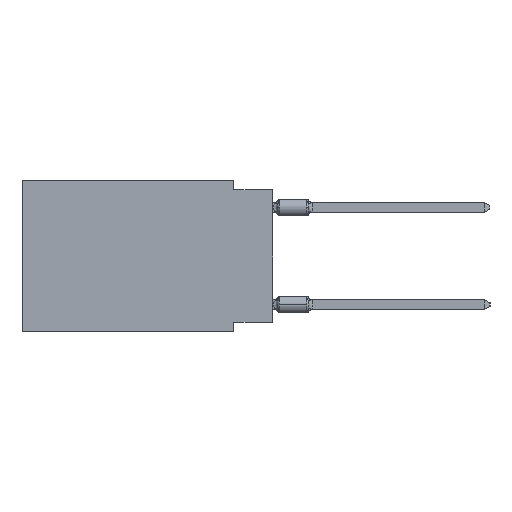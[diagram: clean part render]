
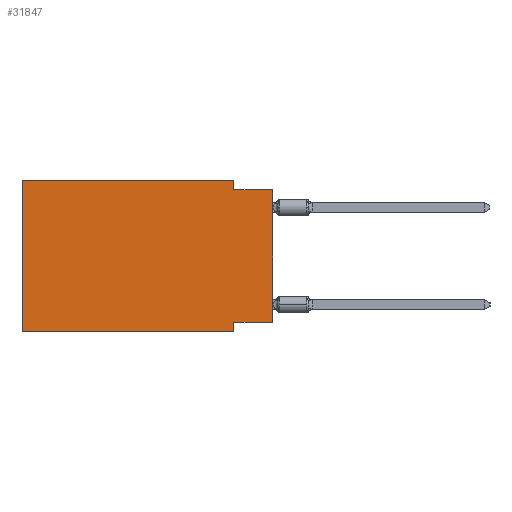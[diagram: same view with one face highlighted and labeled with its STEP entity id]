
A CAD part, left-side view. The second image highlights one B-rep face of the part: STEP entity #31847.
In plain terms, the highlighted planar face has unit normal (-1, 0, 0).
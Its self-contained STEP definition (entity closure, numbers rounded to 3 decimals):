
#620 = CARTESIAN_POINT ( 'NONE',  ( 0., 0., -9.271 ) ) ;
#1028 = VECTOR ( 'NONE', #31118, 1000. ) ;
#1878 = AXIS2_PLACEMENT_3D ( 'NONE', #16112, #35261, #24535 ) ;
#2022 = ORIENTED_EDGE ( 'NONE', *, *, #34639, .F. ) ;
#3643 = CARTESIAN_POINT ( 'NONE',  ( 0., 16.383, 0. ) ) ;
#3653 = VERTEX_POINT ( 'NONE', #5352 ) ;
#4798 = EDGE_CURVE ( 'NONE', #8434, #12249, #26091, .T. ) ;
#5352 = CARTESIAN_POINT ( 'NONE',  ( 0., 0., -9.271 ) ) ;
#5717 = CARTESIAN_POINT ( 'NONE',  ( 0., 2.54, 0. ) ) ;
#5914 = VERTEX_POINT ( 'NONE', #12140 ) ;
#5923 = VECTOR ( 'NONE', #23417, 1000. ) ;
#6857 = EDGE_CURVE ( 'NONE', #8155, #12249, #12496, .T. ) ;
#7357 = VERTEX_POINT ( 'NONE', #21550 ) ;
#7614 = CARTESIAN_POINT ( 'NONE',  ( 0., 16.383, 0. ) ) ;
#8155 = VERTEX_POINT ( 'NONE', #28995 ) ;
#8394 = CARTESIAN_POINT ( 'NONE',  ( 0., 2.54, -9.271 ) ) ;
#8434 = VERTEX_POINT ( 'NONE', #8394 ) ;
#8813 = VECTOR ( 'NONE', #29454, 1000. ) ;
#10159 = EDGE_CURVE ( 'NONE', #3653, #7357, #32649, .T. ) ;
#10333 = VERTEX_POINT ( 'NONE', #3643 ) ;
#11483 = CARTESIAN_POINT ( 'NONE',  ( 0., 2.54, -0.635 ) ) ;
#11567 = ORIENTED_EDGE ( 'NONE', *, *, #13683, .F. ) ;
#12127 = CARTESIAN_POINT ( 'NONE',  ( 0., 16.383, 0. ) ) ;
#12140 = CARTESIAN_POINT ( 'NONE',  ( 0., 2.54, 0. ) ) ;
#12249 = VERTEX_POINT ( 'NONE', #30718 ) ;
#12496 = LINE ( 'NONE', #23749, #5923 ) ;
#12731 = ORIENTED_EDGE ( 'NONE', *, *, #6857, .T. ) ;
#13683 = EDGE_CURVE ( 'NONE', #5914, #21203, #14554, .T. ) ;
#13859 = DIRECTION ( 'NONE',  ( 0., 0., 1. ) ) ;
#14021 = EDGE_CURVE ( 'NONE', #10333, #5914, #17853, .T. ) ;
#14554 = LINE ( 'NONE', #5717, #25412 ) ;
#14580 = VECTOR ( 'NONE', #34665, 1000. ) ;
#14845 = CARTESIAN_POINT ( 'NONE',  ( 0., 2.54, -9.906 ) ) ;
#15474 = ORIENTED_EDGE ( 'NONE', *, *, #4798, .F. ) ;
#16112 = CARTESIAN_POINT ( 'NONE',  ( 0., 16.383, 0. ) ) ;
#16556 = DIRECTION ( 'NONE',  ( 0., 1., 0. ) ) ;
#17853 = LINE ( 'NONE', #12127, #14580 ) ;
#18457 = EDGE_LOOP ( 'NONE', ( #27604, #2022, #11567, #31262, #22287, #12731, #15474, #24645 ) ) ;
#21203 = VERTEX_POINT ( 'NONE', #11483 ) ;
#21550 = CARTESIAN_POINT ( 'NONE',  ( 0., 0., -0.635 ) ) ;
#21902 = CARTESIAN_POINT ( 'NONE',  ( 0., 0., 0. ) ) ;
#21991 = DIRECTION ( 'NONE',  ( 0., 0., -1. ) ) ;
#22287 = ORIENTED_EDGE ( 'NONE', *, *, #28129, .F. ) ;
#23343 = VECTOR ( 'NONE', #25752, 1000. ) ;
#23417 = DIRECTION ( 'NONE',  ( 0., -1., 0. ) ) ;
#23749 = CARTESIAN_POINT ( 'NONE',  ( 0., 16.383, -9.906 ) ) ;
#24535 = DIRECTION ( 'NONE',  ( 0., 0., -1. ) ) ;
#24645 = ORIENTED_EDGE ( 'NONE', *, *, #34885, .F. ) ;
#25080 = VECTOR ( 'NONE', #16556, 1000. ) ;
#25412 = VECTOR ( 'NONE', #21991, 1000. ) ;
#25752 = DIRECTION ( 'NONE',  ( 0., 0., -1. ) ) ;
#26091 = LINE ( 'NONE', #14845, #23343 ) ;
#27604 = ORIENTED_EDGE ( 'NONE', *, *, #10159, .T. ) ;
#27998 = LINE ( 'NONE', #620, #25080 ) ;
#28129 = EDGE_CURVE ( 'NONE', #8155, #10333, #32137, .T. ) ;
#28995 = CARTESIAN_POINT ( 'NONE',  ( 0., 16.383, -9.906 ) ) ;
#29454 = DIRECTION ( 'NONE',  ( 0., 0., 1. ) ) ;
#30607 = VECTOR ( 'NONE', #13859, 1000. ) ;
#30718 = CARTESIAN_POINT ( 'NONE',  ( 0., 2.54, -9.906 ) ) ;
#30951 = CARTESIAN_POINT ( 'NONE',  ( 0., 0., -0.635 ) ) ;
#31118 = DIRECTION ( 'NONE',  ( 0., -1., 0. ) ) ;
#31262 = ORIENTED_EDGE ( 'NONE', *, *, #14021, .F. ) ;
#31847 = ADVANCED_FACE ( 'NONE', ( #34910 ), #32048, .F. ) ;
#32048 = PLANE ( 'NONE',  #1878 ) ;
#32137 = LINE ( 'NONE', #7614, #8813 ) ;
#32649 = LINE ( 'NONE', #21902, #30607 ) ;
#33810 = LINE ( 'NONE', #30951, #1028 ) ;
#34639 = EDGE_CURVE ( 'NONE', #21203, #7357, #33810, .T. ) ;
#34665 = DIRECTION ( 'NONE',  ( 0., -1., 0. ) ) ;
#34885 = EDGE_CURVE ( 'NONE', #3653, #8434, #27998, .T. ) ;
#34910 = FACE_OUTER_BOUND ( 'NONE', #18457, .T. ) ;
#35261 = DIRECTION ( 'NONE',  ( 1., 0., 0. ) ) ;
